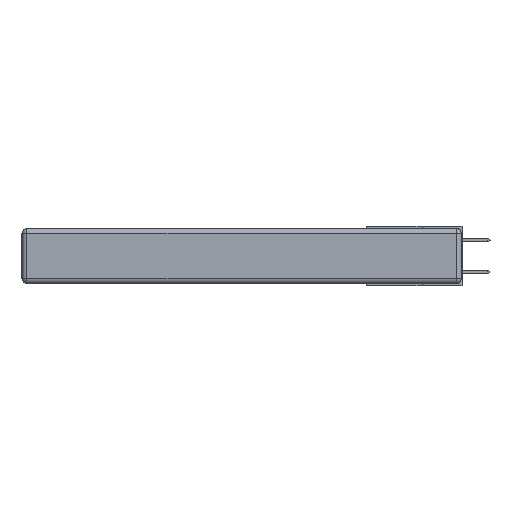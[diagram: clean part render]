
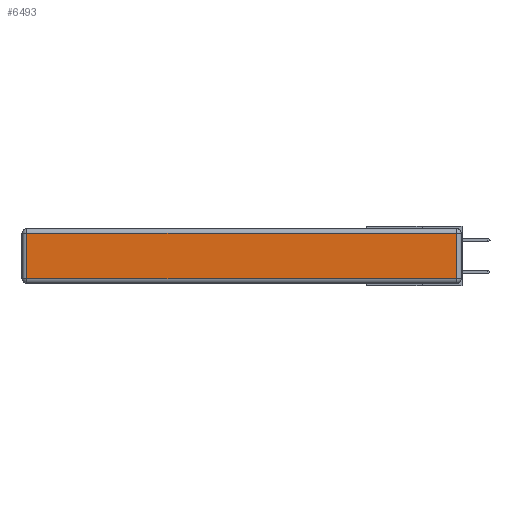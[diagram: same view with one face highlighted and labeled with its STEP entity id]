
A CAD part, left-side view. The second image highlights one B-rep face of the part: STEP entity #6493.
In plain terms, the highlighted planar face has unit normal (-1, 0, 0).
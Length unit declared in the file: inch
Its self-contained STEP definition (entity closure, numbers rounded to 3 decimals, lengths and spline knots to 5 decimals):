
#396 = EDGE_CURVE ( 'NONE', #11733, #20161, #13174, .T. ) ;
#1914 = VERTEX_POINT ( 'NONE', #14812 ) ;
#2528 = DIRECTION ( 'NONE',  ( 0., 1., 0. ) ) ;
#2862 = ORIENTED_EDGE ( 'NONE', *, *, #396, .T. ) ;
#3437 = DIRECTION ( 'NONE',  ( 0., -1., 0. ) ) ;
#4318 = EDGE_LOOP ( 'NONE', ( #5904, #9777, #20178, #2862 ) ) ;
#4890 = CARTESIAN_POINT ( 'NONE',  ( 0., 0., -0.313 ) ) ;
#5904 = ORIENTED_EDGE ( 'NONE', *, *, #14134, .T. ) ;
#6254 = CARTESIAN_POINT ( 'NONE',  ( 0., 0., -0.343 ) ) ;
#6430 = DIRECTION ( 'NONE',  ( 0., 0., 1. ) ) ;
#6493 = ADVANCED_FACE ( 'NONE', ( #8919 ), #14259, .T. ) ;
#6659 = AXIS2_PLACEMENT_3D ( 'NONE', #6254, #7883, #19036 ) ;
#7883 = DIRECTION ( 'NONE',  ( -1., 0., 0. ) ) ;
#7953 = LINE ( 'NONE', #12061, #13647 ) ;
#8841 = VERTEX_POINT ( 'NONE', #13139 ) ;
#8919 = FACE_OUTER_BOUND ( 'NONE', #4318, .T. ) ;
#9049 = CARTESIAN_POINT ( 'NONE',  ( 0., 2.72, -0.03 ) ) ;
#9777 = ORIENTED_EDGE ( 'NONE', *, *, #10724, .T. ) ;
#10008 = LINE ( 'NONE', #19353, #14212 ) ;
#10724 = EDGE_CURVE ( 'NONE', #1914, #8841, #10008, .T. ) ;
#11087 = VECTOR ( 'NONE', #3437, 39.37008 ) ;
#11733 = VERTEX_POINT ( 'NONE', #9049 ) ;
#12061 = CARTESIAN_POINT ( 'NONE',  ( 0., 2.75, -0.03 ) ) ;
#12833 = CARTESIAN_POINT ( 'NONE',  ( 0., 2.72, -0.343 ) ) ;
#13139 = CARTESIAN_POINT ( 'NONE',  ( 0., 0.03, -0.03 ) ) ;
#13174 = LINE ( 'NONE', #12833, #14691 ) ;
#13327 = LINE ( 'NONE', #4890, #11087 ) ;
#13647 = VECTOR ( 'NONE', #2528, 39.37008 ) ;
#14134 = EDGE_CURVE ( 'NONE', #20161, #1914, #13327, .T. ) ;
#14212 = VECTOR ( 'NONE', #6430, 39.37008 ) ;
#14259 = PLANE ( 'NONE',  #6659 ) ;
#14691 = VECTOR ( 'NONE', #15985, 39.37008 ) ;
#14812 = CARTESIAN_POINT ( 'NONE',  ( 0., 0.03, -0.313 ) ) ;
#15985 = DIRECTION ( 'NONE',  ( 0., 0., -1. ) ) ;
#19036 = DIRECTION ( 'NONE',  ( 0., 0., 1. ) ) ;
#19353 = CARTESIAN_POINT ( 'NONE',  ( 0., 0.03, -0.343 ) ) ;
#19530 = CARTESIAN_POINT ( 'NONE',  ( 0., 2.72, -0.313 ) ) ;
#19833 = EDGE_CURVE ( 'NONE', #8841, #11733, #7953, .T. ) ;
#20161 = VERTEX_POINT ( 'NONE', #19530 ) ;
#20178 = ORIENTED_EDGE ( 'NONE', *, *, #19833, .T. ) ;
